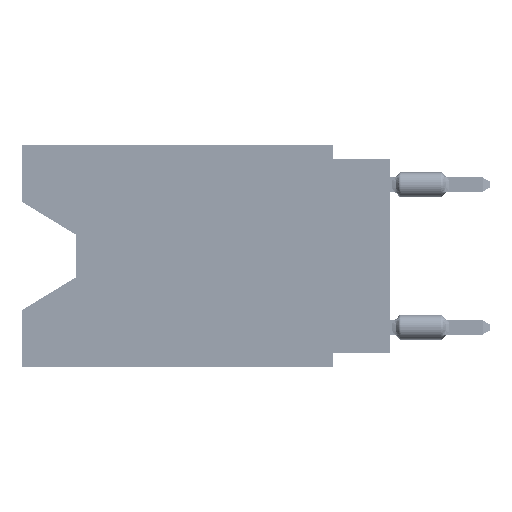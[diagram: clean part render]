
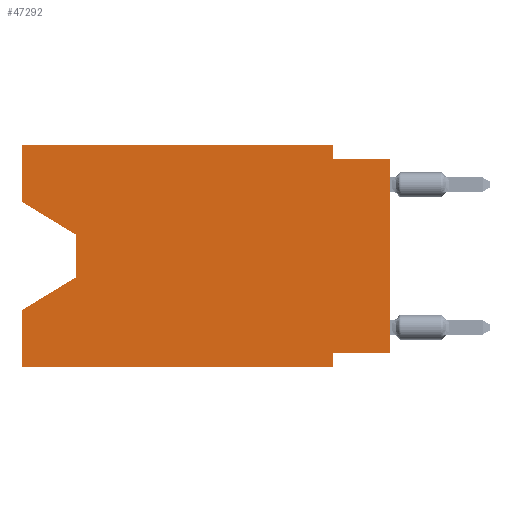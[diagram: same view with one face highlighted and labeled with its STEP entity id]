
A CAD part, left-side view. The second image highlights one B-rep face of the part: STEP entity #47292.
In plain terms, the highlighted planar face has unit normal (-1, 0, 0).
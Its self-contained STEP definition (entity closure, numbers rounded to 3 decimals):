
#896 = LINE ( 'NONE', #1772, #45020 ) ;
#1604 = DIRECTION ( 'NONE',  ( 0., 1., 0. ) ) ;
#1768 = VECTOR ( 'NONE', #43772, 1000. ) ;
#1772 = CARTESIAN_POINT ( 'NONE',  ( 0., 13.97, -4.013 ) ) ;
#2611 = LINE ( 'NONE', #16107, #13588 ) ;
#3069 = LINE ( 'NONE', #28915, #11509 ) ;
#3351 = EDGE_LOOP ( 'NONE', ( #56215, #29092, #56283, #30133, #5043, #12593, #19386, #33481, #35992, #39595, #49131, #44955 ) ) ;
#3484 = CARTESIAN_POINT ( 'NONE',  ( 0., 2.54, 0. ) ) ;
#4842 = LINE ( 'NONE', #52051, #18939 ) ;
#5043 = ORIENTED_EDGE ( 'NONE', *, *, #31325, .T. ) ;
#5607 = CARTESIAN_POINT ( 'NONE',  ( 0., 0., -9.271 ) ) ;
#6688 = DIRECTION ( 'NONE',  ( 0., 0.855, -0.519 ) ) ;
#7143 = DIRECTION ( 'NONE',  ( 0., -1., 0. ) ) ;
#7303 = DIRECTION ( 'NONE',  ( 0., 0., 1. ) ) ;
#7919 = VERTEX_POINT ( 'NONE', #38801 ) ;
#8375 = VERTEX_POINT ( 'NONE', #21963 ) ;
#8450 = CARTESIAN_POINT ( 'NONE',  ( 0., 2.54, -9.906 ) ) ;
#8810 = EDGE_CURVE ( 'NONE', #51599, #43443, #896, .T. ) ;
#9814 = EDGE_CURVE ( 'NONE', #17365, #37453, #10723, .T. ) ;
#10723 = LINE ( 'NONE', #28634, #27732 ) ;
#11139 = VECTOR ( 'NONE', #23453, 1000. ) ;
#11509 = VECTOR ( 'NONE', #39151, 1000. ) ;
#12593 = ORIENTED_EDGE ( 'NONE', *, *, #38485, .F. ) ;
#13476 = VECTOR ( 'NONE', #18837, 1000. ) ;
#13588 = VECTOR ( 'NONE', #7303, 1000. ) ;
#15275 = EDGE_CURVE ( 'NONE', #55694, #7919, #16484, .T. ) ;
#15279 = AXIS2_PLACEMENT_3D ( 'NONE', #49116, #35032, #52944 ) ;
#16107 = CARTESIAN_POINT ( 'NONE',  ( 0., 16.383, 0. ) ) ;
#16447 = LINE ( 'NONE', #24671, #40663 ) ;
#16484 = LINE ( 'NONE', #43203, #1768 ) ;
#17365 = VERTEX_POINT ( 'NONE', #5607 ) ;
#18791 = DIRECTION ( 'NONE',  ( 0., 0., -1. ) ) ;
#18837 = DIRECTION ( 'NONE',  ( 0., 0., 1. ) ) ;
#18939 = VECTOR ( 'NONE', #7143, 1000. ) ;
#19386 = ORIENTED_EDGE ( 'NONE', *, *, #47030, .F. ) ;
#19861 = CARTESIAN_POINT ( 'NONE',  ( 0., 13.97, -4.013 ) ) ;
#20586 = EDGE_CURVE ( 'NONE', #43443, #20947, #46892, .T. ) ;
#20947 = VERTEX_POINT ( 'NONE', #54019 ) ;
#21658 = CARTESIAN_POINT ( 'NONE',  ( 0., 16.383, 0. ) ) ;
#21963 = CARTESIAN_POINT ( 'NONE',  ( 0., 16.383, -9.906 ) ) ;
#23453 = DIRECTION ( 'NONE',  ( 0., -1., 0. ) ) ;
#24671 = CARTESIAN_POINT ( 'NONE',  ( 0., 16.383, -2.546 ) ) ;
#26333 = VERTEX_POINT ( 'NONE', #33350 ) ;
#27727 = CARTESIAN_POINT ( 'NONE',  ( 0., 0., -9.271 ) ) ;
#27732 = VECTOR ( 'NONE', #28345, 1000. ) ;
#28345 = DIRECTION ( 'NONE',  ( 0., 0., 1. ) ) ;
#28634 = CARTESIAN_POINT ( 'NONE',  ( 0., 0., 0. ) ) ;
#28915 = CARTESIAN_POINT ( 'NONE',  ( 0., 16.383, 0. ) ) ;
#29092 = ORIENTED_EDGE ( 'NONE', *, *, #8810, .T. ) ;
#30133 = ORIENTED_EDGE ( 'NONE', *, *, #48295, .F. ) ;
#30764 = DIRECTION ( 'NONE',  ( 0., 0., -1. ) ) ;
#31325 = EDGE_CURVE ( 'NONE', #8375, #26333, #4842, .T. ) ;
#31940 = CARTESIAN_POINT ( 'NONE',  ( 0., 16.383, 0. ) ) ;
#32273 = LINE ( 'NONE', #50472, #11139 ) ;
#33350 = CARTESIAN_POINT ( 'NONE',  ( 0., 2.54, -9.906 ) ) ;
#33481 = ORIENTED_EDGE ( 'NONE', *, *, #9814, .T. ) ;
#35032 = DIRECTION ( 'NONE',  ( 1., 0., 0. ) ) ;
#35811 = CARTESIAN_POINT ( 'NONE',  ( 0., 2.54, -9.271 ) ) ;
#35992 = ORIENTED_EDGE ( 'NONE', *, *, #55570, .F. ) ;
#36355 = VERTEX_POINT ( 'NONE', #35811 ) ;
#37221 = CARTESIAN_POINT ( 'NONE',  ( 0., 16.383, -2.546 ) ) ;
#37453 = VERTEX_POINT ( 'NONE', #55291 ) ;
#38485 = EDGE_CURVE ( 'NONE', #36355, #26333, #57754, .T. ) ;
#38801 = CARTESIAN_POINT ( 'NONE',  ( 0., 2.54, -0.635 ) ) ;
#39151 = DIRECTION ( 'NONE',  ( 0., -1., 0. ) ) ;
#39595 = ORIENTED_EDGE ( 'NONE', *, *, #15275, .F. ) ;
#40663 = VECTOR ( 'NONE', #43163, 1000. ) ;
#41245 = CARTESIAN_POINT ( 'NONE',  ( 0., 13.97, -5.893 ) ) ;
#41812 = LINE ( 'NONE', #27727, #53801 ) ;
#42763 = CARTESIAN_POINT ( 'NONE',  ( 0., 13.97, -5.893 ) ) ;
#43163 = DIRECTION ( 'NONE',  ( 0., -0.855, -0.519 ) ) ;
#43203 = CARTESIAN_POINT ( 'NONE',  ( 0., 2.54, 0. ) ) ;
#43443 = VERTEX_POINT ( 'NONE', #41245 ) ;
#43772 = DIRECTION ( 'NONE',  ( 0., 0., -1. ) ) ;
#44695 = PLANE ( 'NONE',  #15279 ) ;
#44955 = ORIENTED_EDGE ( 'NONE', *, *, #50068, .F. ) ;
#45020 = VECTOR ( 'NONE', #18791, 1000. ) ;
#45109 = VECTOR ( 'NONE', #6688, 1000. ) ;
#46257 = VERTEX_POINT ( 'NONE', #21658 ) ;
#46892 = LINE ( 'NONE', #42763, #45109 ) ;
#47030 = EDGE_CURVE ( 'NONE', #17365, #36355, #41812, .T. ) ;
#47146 = EDGE_CURVE ( 'NONE', #46257, #55694, #3069, .T. ) ;
#47292 = ADVANCED_FACE ( 'NONE', ( #48822 ), #44695, .F. ) ;
#48295 = EDGE_CURVE ( 'NONE', #8375, #20947, #54244, .T. ) ;
#48537 = EDGE_CURVE ( 'NONE', #57724, #51599, #16447, .T. ) ;
#48822 = FACE_OUTER_BOUND ( 'NONE', #3351, .T. ) ;
#49116 = CARTESIAN_POINT ( 'NONE',  ( 0., 16.383, 0. ) ) ;
#49131 = ORIENTED_EDGE ( 'NONE', *, *, #47146, .F. ) ;
#50068 = EDGE_CURVE ( 'NONE', #57724, #46257, #2611, .T. ) ;
#50472 = CARTESIAN_POINT ( 'NONE',  ( 0., 0., -0.635 ) ) ;
#51271 = VECTOR ( 'NONE', #30764, 1000. ) ;
#51599 = VERTEX_POINT ( 'NONE', #19861 ) ;
#52051 = CARTESIAN_POINT ( 'NONE',  ( 0., 16.383, -9.906 ) ) ;
#52944 = DIRECTION ( 'NONE',  ( 0., 0., -1. ) ) ;
#53801 = VECTOR ( 'NONE', #1604, 1000. ) ;
#54019 = CARTESIAN_POINT ( 'NONE',  ( 0., 16.383, -7.36 ) ) ;
#54244 = LINE ( 'NONE', #31940, #13476 ) ;
#55291 = CARTESIAN_POINT ( 'NONE',  ( 0., 0., -0.635 ) ) ;
#55570 = EDGE_CURVE ( 'NONE', #7919, #37453, #32273, .T. ) ;
#55694 = VERTEX_POINT ( 'NONE', #3484 ) ;
#56215 = ORIENTED_EDGE ( 'NONE', *, *, #48537, .T. ) ;
#56283 = ORIENTED_EDGE ( 'NONE', *, *, #20586, .T. ) ;
#57724 = VERTEX_POINT ( 'NONE', #37221 ) ;
#57754 = LINE ( 'NONE', #8450, #51271 ) ;
